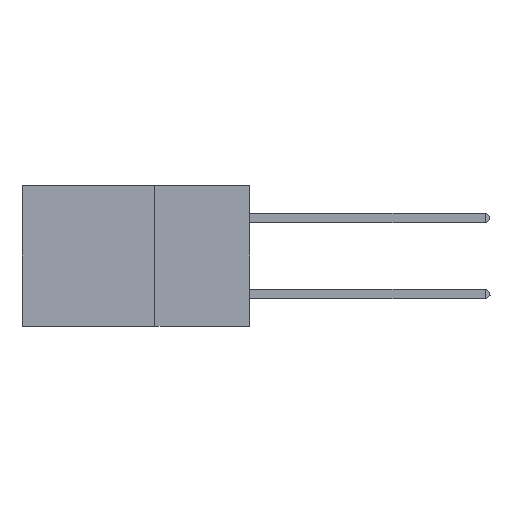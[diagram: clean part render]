
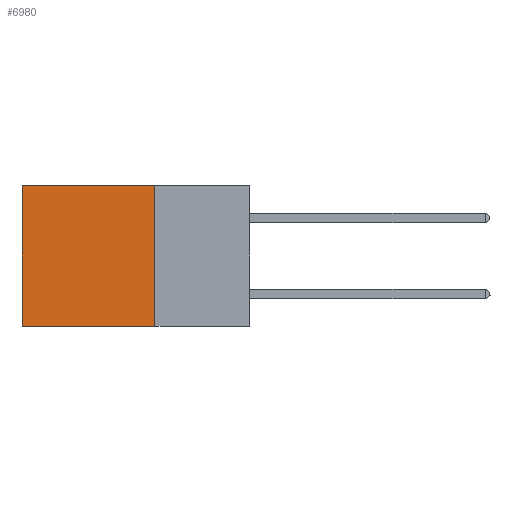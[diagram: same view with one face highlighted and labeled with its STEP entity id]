
A CAD part, left-side view. The second image highlights one B-rep face of the part: STEP entity #6980.
In plain terms, the highlighted planar face has unit normal (-1, 0, 0).
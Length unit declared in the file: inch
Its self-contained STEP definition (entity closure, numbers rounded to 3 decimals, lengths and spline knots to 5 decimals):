
#267 = VECTOR ( 'NONE', #14354, 39.37008 ) ;
#1252 = VERTEX_POINT ( 'NONE', #25717 ) ;
#4009 = CARTESIAN_POINT ( 'NONE',  ( 0.2875, 0.25, 0. ) ) ;
#4282 = ORIENTED_EDGE ( 'NONE', *, *, #34102, .F. ) ;
#6319 = CARTESIAN_POINT ( 'NONE',  ( 0.2875, 0.25, 0. ) ) ;
#6980 = ADVANCED_FACE ( 'NONE', ( #26975 ), #32057, .F. ) ;
#8896 = EDGE_LOOP ( 'NONE', ( #20378, #4282, #31319, #40177 ) ) ;
#9211 = EDGE_CURVE ( 'NONE', #27896, #33970, #38012, .T. ) ;
#14209 = DIRECTION ( 'NONE',  ( 0., 0., -1. ) ) ;
#14354 = DIRECTION ( 'NONE',  ( 0., 1., 0. ) ) ;
#15312 = VECTOR ( 'NONE', #20315, 39.37008 ) ;
#15433 = EDGE_CURVE ( 'NONE', #1252, #26591, #36669, .T. ) ;
#15572 = DIRECTION ( 'NONE',  ( 1., 0., 0. ) ) ;
#15820 = CARTESIAN_POINT ( 'NONE',  ( 0.2875, 0.6, -0.37 ) ) ;
#17054 = CARTESIAN_POINT ( 'NONE',  ( 0.2875, 0.6, 0. ) ) ;
#17125 = VECTOR ( 'NONE', #14209, 39.37008 ) ;
#17397 = EDGE_CURVE ( 'NONE', #27896, #1252, #17541, .T. ) ;
#17541 = LINE ( 'NONE', #40209, #267 ) ;
#18641 = VECTOR ( 'NONE', #37223, 39.37008 ) ;
#20315 = DIRECTION ( 'NONE',  ( 0., 0., -1. ) ) ;
#20378 = ORIENTED_EDGE ( 'NONE', *, *, #15433, .T. ) ;
#20875 = CARTESIAN_POINT ( 'NONE',  ( 0.2875, 0.25, -0.37 ) ) ;
#22114 = DIRECTION ( 'NONE',  ( 0., 0., -1. ) ) ;
#25717 = CARTESIAN_POINT ( 'NONE',  ( 0.2875, 0.6, 0. ) ) ;
#26591 = VERTEX_POINT ( 'NONE', #15820 ) ;
#26975 = FACE_OUTER_BOUND ( 'NONE', #8896, .T. ) ;
#27896 = VERTEX_POINT ( 'NONE', #41449 ) ;
#31319 = ORIENTED_EDGE ( 'NONE', *, *, #9211, .F. ) ;
#32057 = PLANE ( 'NONE',  #34923 ) ;
#33276 = CARTESIAN_POINT ( 'NONE',  ( 0.2875, 0.25, -0.37 ) ) ;
#33970 = VERTEX_POINT ( 'NONE', #33276 ) ;
#34102 = EDGE_CURVE ( 'NONE', #33970, #26591, #35403, .T. ) ;
#34923 = AXIS2_PLACEMENT_3D ( 'NONE', #6319, #15572, #22114 ) ;
#35403 = LINE ( 'NONE', #20875, #18641 ) ;
#36669 = LINE ( 'NONE', #17054, #15312 ) ;
#37223 = DIRECTION ( 'NONE',  ( 0., 1., 0. ) ) ;
#38012 = LINE ( 'NONE', #4009, #17125 ) ;
#40177 = ORIENTED_EDGE ( 'NONE', *, *, #17397, .T. ) ;
#40209 = CARTESIAN_POINT ( 'NONE',  ( 0.2875, 0.25, 0. ) ) ;
#41449 = CARTESIAN_POINT ( 'NONE',  ( 0.2875, 0.25, 0. ) ) ;
